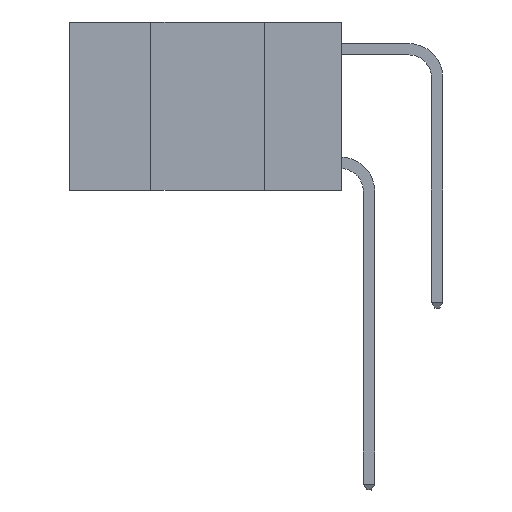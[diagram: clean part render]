
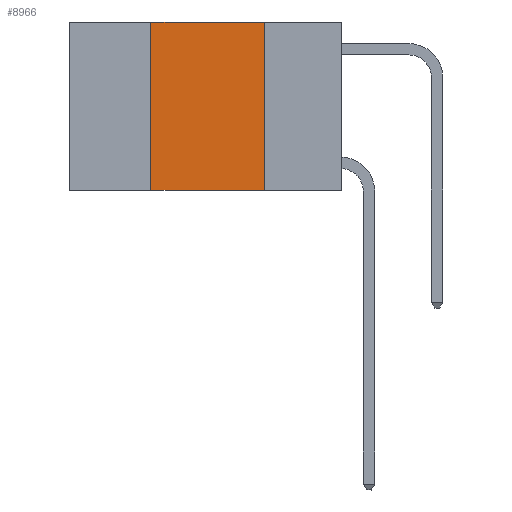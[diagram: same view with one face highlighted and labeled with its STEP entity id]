
A CAD part, left-side view. The second image highlights one B-rep face of the part: STEP entity #8966.
In plain terms, the highlighted planar face has unit normal (-1, 0, 0).
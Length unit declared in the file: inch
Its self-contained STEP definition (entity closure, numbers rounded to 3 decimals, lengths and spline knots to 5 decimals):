
#255 = VERTEX_POINT ( 'NONE', #10586 ) ;
#275 = VERTEX_POINT ( 'NONE', #3592 ) ;
#683 = ORIENTED_EDGE ( 'NONE', *, *, #6063, .T. ) ;
#836 = CARTESIAN_POINT ( 'NONE',  ( 0., 0.17, -0.37 ) ) ;
#1274 = VECTOR ( 'NONE', #1581, 39.37008 ) ;
#1450 = DIRECTION ( 'NONE',  ( 0., 0., -1. ) ) ;
#1454 = ORIENTED_EDGE ( 'NONE', *, *, #1706, .F. ) ;
#1581 = DIRECTION ( 'NONE',  ( 0., 0., -1. ) ) ;
#1706 = EDGE_CURVE ( 'NONE', #2899, #9477, #5924, .T. ) ;
#2385 = EDGE_CURVE ( 'NONE', #275, #255, #8764, .T. ) ;
#2870 = LINE ( 'NONE', #11020, #8173 ) ;
#2899 = VERTEX_POINT ( 'NONE', #6781 ) ;
#3016 = CARTESIAN_POINT ( 'NONE',  ( 0., 0.17, 0. ) ) ;
#3422 = DIRECTION ( 'NONE',  ( 0., -1., 0. ) ) ;
#3592 = CARTESIAN_POINT ( 'NONE',  ( 0., 0.42, -0.37 ) ) ;
#3961 = DIRECTION ( 'NONE',  ( 1., 0., 0. ) ) ;
#3971 = AXIS2_PLACEMENT_3D ( 'NONE', #4924, #3961, #1450 ) ;
#4911 = CARTESIAN_POINT ( 'NONE',  ( 0., 0.6, -0.37 ) ) ;
#4924 = CARTESIAN_POINT ( 'NONE',  ( 0., 0.6, 0. ) ) ;
#5179 = EDGE_LOOP ( 'NONE', ( #1454, #8734, #10234, #683 ) ) ;
#5924 = LINE ( 'NONE', #3016, #1274 ) ;
#6063 = EDGE_CURVE ( 'NONE', #275, #9477, #10479, .T. ) ;
#6376 = VECTOR ( 'NONE', #8645, 39.37008 ) ;
#6781 = CARTESIAN_POINT ( 'NONE',  ( 0., 0.17, 0. ) ) ;
#7044 = CARTESIAN_POINT ( 'NONE',  ( 0., 0.42, 0. ) ) ;
#7986 = EDGE_CURVE ( 'NONE', #255, #2899, #2870, .T. ) ;
#8058 = VECTOR ( 'NONE', #3422, 39.37008 ) ;
#8173 = VECTOR ( 'NONE', #10049, 39.37008 ) ;
#8645 = DIRECTION ( 'NONE',  ( 0., 0., 1. ) ) ;
#8734 = ORIENTED_EDGE ( 'NONE', *, *, #7986, .F. ) ;
#8764 = LINE ( 'NONE', #7044, #6376 ) ;
#8966 = ADVANCED_FACE ( 'NONE', ( #11130 ), #9485, .F. ) ;
#9477 = VERTEX_POINT ( 'NONE', #836 ) ;
#9485 = PLANE ( 'NONE',  #3971 ) ;
#10049 = DIRECTION ( 'NONE',  ( 0., -1., 0. ) ) ;
#10234 = ORIENTED_EDGE ( 'NONE', *, *, #2385, .F. ) ;
#10479 = LINE ( 'NONE', #4911, #8058 ) ;
#10586 = CARTESIAN_POINT ( 'NONE',  ( 0., 0.42, 0. ) ) ;
#11020 = CARTESIAN_POINT ( 'NONE',  ( 0., 0.6, 0. ) ) ;
#11130 = FACE_OUTER_BOUND ( 'NONE', #5179, .T. ) ;
